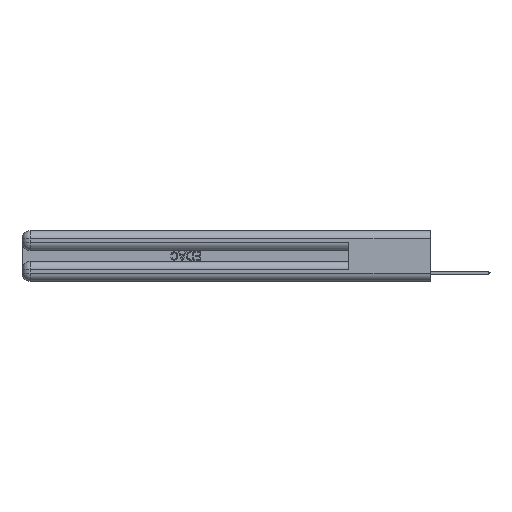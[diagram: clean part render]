
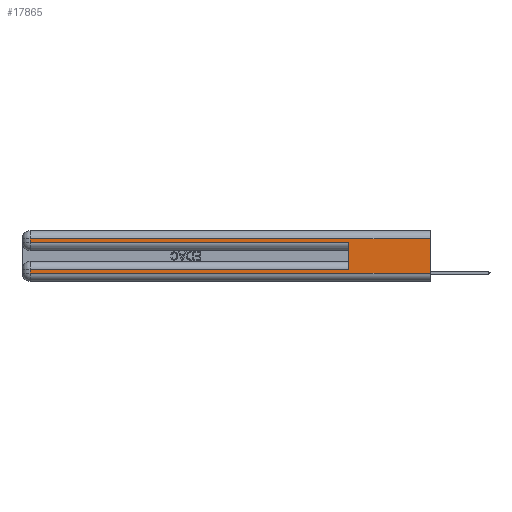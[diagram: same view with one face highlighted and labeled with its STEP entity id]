
A CAD part, left-side view. The second image highlights one B-rep face of the part: STEP entity #17865.
In plain terms, the highlighted planar face has unit normal (-1, 0, 0).
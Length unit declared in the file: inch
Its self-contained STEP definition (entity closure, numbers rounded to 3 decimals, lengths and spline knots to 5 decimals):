
#277 = EDGE_CURVE ( 'NONE', #17744, #21540, #12206, .T. ) ;
#538 = CARTESIAN_POINT ( 'NONE',  ( 0., 0., 0.06 ) ) ;
#753 = CARTESIAN_POINT ( 'NONE',  ( 0., 2.94, 0.37 ) ) ;
#1882 = DIRECTION ( 'NONE',  ( 0., 0., -1. ) ) ;
#2205 = VERTEX_POINT ( 'NONE', #17006 ) ;
#2258 = VECTOR ( 'NONE', #31003, 39.37008 ) ;
#2354 = CARTESIAN_POINT ( 'NONE',  ( 0., 2.94, 0.31 ) ) ;
#2775 = DIRECTION ( 'NONE',  ( 0., 0., 1. ) ) ;
#3725 = FACE_OUTER_BOUND ( 'NONE', #30161, .T. ) ;
#4177 = VECTOR ( 'NONE', #21189, 39.37008 ) ;
#4334 = LINE ( 'NONE', #4850, #18621 ) ;
#4409 = VERTEX_POINT ( 'NONE', #29944 ) ;
#4850 = CARTESIAN_POINT ( 'NONE',  ( 0., 0., 0.285 ) ) ;
#5084 = DIRECTION ( 'NONE',  ( 0., -1., 0. ) ) ;
#5372 = AXIS2_PLACEMENT_3D ( 'NONE', #20613, #25789, #1882 ) ;
#5466 = LINE ( 'NONE', #18360, #8882 ) ;
#6091 = CARTESIAN_POINT ( 'NONE',  ( 0., 0.6, 0.085 ) ) ;
#6715 = ORIENTED_EDGE ( 'NONE', *, *, #8991, .T. ) ;
#7328 = VERTEX_POINT ( 'NONE', #9165 ) ;
#7347 = ORIENTED_EDGE ( 'NONE', *, *, #10250, .F. ) ;
#8882 = VECTOR ( 'NONE', #16216, 39.37008 ) ;
#8991 = EDGE_CURVE ( 'NONE', #20948, #16314, #24043, .T. ) ;
#9026 = LINE ( 'NONE', #17917, #20728 ) ;
#9165 = CARTESIAN_POINT ( 'NONE',  ( 0., 2.94, 0.285 ) ) ;
#9959 = DIRECTION ( 'NONE',  ( 0., 0., -1. ) ) ;
#10148 = EDGE_CURVE ( 'NONE', #2205, #21540, #27914, .T. ) ;
#10250 = EDGE_CURVE ( 'NONE', #20948, #4409, #17114, .T. ) ;
#10398 = EDGE_CURVE ( 'NONE', #16314, #2205, #23526, .T. ) ;
#11249 = VERTEX_POINT ( 'NONE', #2354 ) ;
#11932 = ORIENTED_EDGE ( 'NONE', *, *, #31217, .T. ) ;
#12032 = ORIENTED_EDGE ( 'NONE', *, *, #10148, .T. ) ;
#12206 = LINE ( 'NONE', #26483, #4177 ) ;
#14310 = PLANE ( 'NONE',  #5372 ) ;
#14908 = ORIENTED_EDGE ( 'NONE', *, *, #20672, .T. ) ;
#14956 = CARTESIAN_POINT ( 'NONE',  ( 0., 0., 0.085 ) ) ;
#15003 = VECTOR ( 'NONE', #2775, 39.37008 ) ;
#15499 = EDGE_CURVE ( 'NONE', #7328, #4409, #4334, .T. ) ;
#16216 = DIRECTION ( 'NONE',  ( 0., 1., 0. ) ) ;
#16314 = VERTEX_POINT ( 'NONE', #23309 ) ;
#17006 = CARTESIAN_POINT ( 'NONE',  ( 0., 2.94, 0.06 ) ) ;
#17114 = LINE ( 'NONE', #24447, #15003 ) ;
#17744 = VERTEX_POINT ( 'NONE', #21669 ) ;
#17865 = ADVANCED_FACE ( 'NONE', ( #3725 ), #14310, .F. ) ;
#17917 = CARTESIAN_POINT ( 'NONE',  ( 0., 2.94, 0.37 ) ) ;
#18259 = CARTESIAN_POINT ( 'NONE',  ( 0., 0., 0.06 ) ) ;
#18360 = CARTESIAN_POINT ( 'NONE',  ( 0., 0., 0.31 ) ) ;
#18621 = VECTOR ( 'NONE', #31943, 39.37008 ) ;
#20613 = CARTESIAN_POINT ( 'NONE',  ( 0., 0., 0.37 ) ) ;
#20672 = EDGE_CURVE ( 'NONE', #11249, #7328, #9026, .T. ) ;
#20728 = VECTOR ( 'NONE', #9959, 39.37008 ) ;
#20948 = VERTEX_POINT ( 'NONE', #6091 ) ;
#21189 = DIRECTION ( 'NONE',  ( 0., 0., -1. ) ) ;
#21540 = VERTEX_POINT ( 'NONE', #538 ) ;
#21669 = CARTESIAN_POINT ( 'NONE',  ( 0., 0., 0.31 ) ) ;
#22600 = ORIENTED_EDGE ( 'NONE', *, *, #277, .F. ) ;
#23309 = CARTESIAN_POINT ( 'NONE',  ( 0., 2.94, 0.085 ) ) ;
#23526 = LINE ( 'NONE', #753, #32322 ) ;
#24043 = LINE ( 'NONE', #14956, #2258 ) ;
#24447 = CARTESIAN_POINT ( 'NONE',  ( 0., 0.6, 0.145 ) ) ;
#24960 = ORIENTED_EDGE ( 'NONE', *, *, #10398, .T. ) ;
#25789 = DIRECTION ( 'NONE',  ( 1., 0., 0. ) ) ;
#26483 = CARTESIAN_POINT ( 'NONE',  ( 0., 0., 0.37 ) ) ;
#26574 = ORIENTED_EDGE ( 'NONE', *, *, #15499, .T. ) ;
#27914 = LINE ( 'NONE', #18259, #31687 ) ;
#29937 = DIRECTION ( 'NONE',  ( 0., 0., -1. ) ) ;
#29944 = CARTESIAN_POINT ( 'NONE',  ( 0., 0.6, 0.285 ) ) ;
#30161 = EDGE_LOOP ( 'NONE', ( #22600, #11932, #14908, #26574, #7347, #6715, #24960, #12032 ) ) ;
#31003 = DIRECTION ( 'NONE',  ( 0., 1., 0. ) ) ;
#31217 = EDGE_CURVE ( 'NONE', #17744, #11249, #5466, .T. ) ;
#31687 = VECTOR ( 'NONE', #5084, 39.37008 ) ;
#31943 = DIRECTION ( 'NONE',  ( 0., -1., 0. ) ) ;
#32322 = VECTOR ( 'NONE', #29937, 39.37008 ) ;
